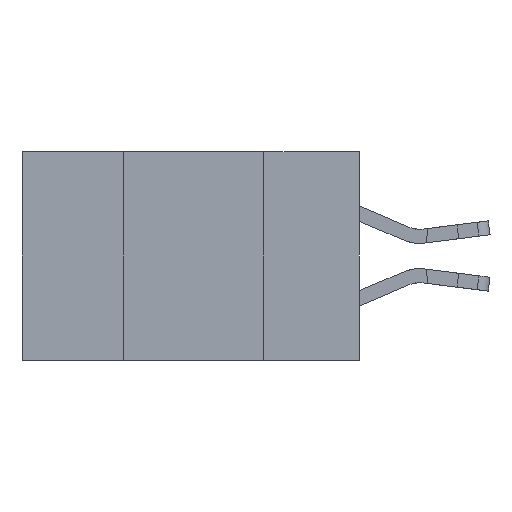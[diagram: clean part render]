
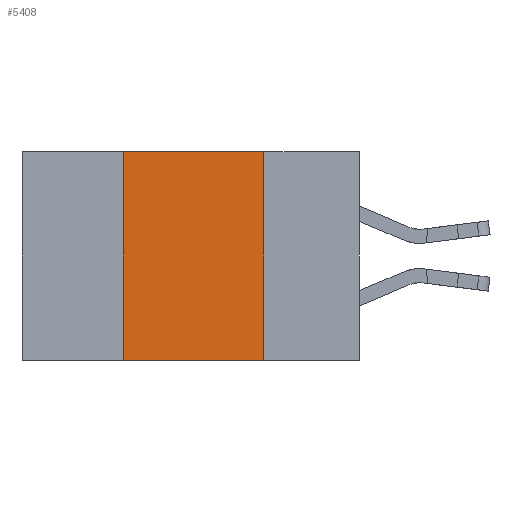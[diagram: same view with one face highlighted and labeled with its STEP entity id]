
A CAD part, left-side view. The second image highlights one B-rep face of the part: STEP entity #5408.
In plain terms, the highlighted planar face has unit normal (-1, 0, 0).
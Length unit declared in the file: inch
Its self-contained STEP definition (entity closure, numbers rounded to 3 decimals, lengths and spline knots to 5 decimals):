
#439 = LINE ( 'NONE', #17493, #10171 ) ;
#764 = DIRECTION ( 'NONE',  ( 0., 0., -1. ) ) ;
#930 = VECTOR ( 'NONE', #2016, 39.37008 ) ;
#1289 = EDGE_CURVE ( 'NONE', #5376, #19676, #14821, .T. ) ;
#1799 = CARTESIAN_POINT ( 'NONE',  ( 0., 0.42, -0.37 ) ) ;
#1995 = EDGE_LOOP ( 'NONE', ( #7376, #12566, #13175, #13764 ) ) ;
#2016 = DIRECTION ( 'NONE',  ( 0., 0., 1. ) ) ;
#3562 = EDGE_CURVE ( 'NONE', #7690, #19676, #439, .T. ) ;
#3721 = VECTOR ( 'NONE', #5712, 39.37008 ) ;
#4804 = FACE_OUTER_BOUND ( 'NONE', #1995, .T. ) ;
#5083 = DIRECTION ( 'NONE',  ( 1., 0., 0. ) ) ;
#5133 = DIRECTION ( 'NONE',  ( 0., 0., -1. ) ) ;
#5376 = VERTEX_POINT ( 'NONE', #17569 ) ;
#5408 = ADVANCED_FACE ( 'NONE', ( #4804 ), #18074, .F. ) ;
#5712 = DIRECTION ( 'NONE',  ( 0., -1., 0. ) ) ;
#5974 = CARTESIAN_POINT ( 'NONE',  ( 0., 0.42, 0. ) ) ;
#7376 = ORIENTED_EDGE ( 'NONE', *, *, #1289, .F. ) ;
#7690 = VERTEX_POINT ( 'NONE', #1799 ) ;
#8330 = EDGE_CURVE ( 'NONE', #17565, #5376, #8908, .T. ) ;
#8908 = LINE ( 'NONE', #11477, #3721 ) ;
#10171 = VECTOR ( 'NONE', #16277, 39.37008 ) ;
#11477 = CARTESIAN_POINT ( 'NONE',  ( 0., 0.6, 0. ) ) ;
#11767 = CARTESIAN_POINT ( 'NONE',  ( 0., 0.6, 0. ) ) ;
#12566 = ORIENTED_EDGE ( 'NONE', *, *, #8330, .F. ) ;
#12998 = CARTESIAN_POINT ( 'NONE',  ( 0., 0.17, -0.37 ) ) ;
#13175 = ORIENTED_EDGE ( 'NONE', *, *, #17386, .F. ) ;
#13764 = ORIENTED_EDGE ( 'NONE', *, *, #3562, .T. ) ;
#14821 = LINE ( 'NONE', #22605, #19302 ) ;
#16277 = DIRECTION ( 'NONE',  ( 0., -1., 0. ) ) ;
#17386 = EDGE_CURVE ( 'NONE', #7690, #17565, #21473, .T. ) ;
#17493 = CARTESIAN_POINT ( 'NONE',  ( 0., 0.6, -0.37 ) ) ;
#17565 = VERTEX_POINT ( 'NONE', #18249 ) ;
#17569 = CARTESIAN_POINT ( 'NONE',  ( 0., 0.17, 0. ) ) ;
#18074 = PLANE ( 'NONE',  #19142 ) ;
#18249 = CARTESIAN_POINT ( 'NONE',  ( 0., 0.42, 0. ) ) ;
#19142 = AXIS2_PLACEMENT_3D ( 'NONE', #11767, #5083, #764 ) ;
#19302 = VECTOR ( 'NONE', #5133, 39.37008 ) ;
#19676 = VERTEX_POINT ( 'NONE', #12998 ) ;
#21473 = LINE ( 'NONE', #5974, #930 ) ;
#22605 = CARTESIAN_POINT ( 'NONE',  ( 0., 0.17, 0. ) ) ;
